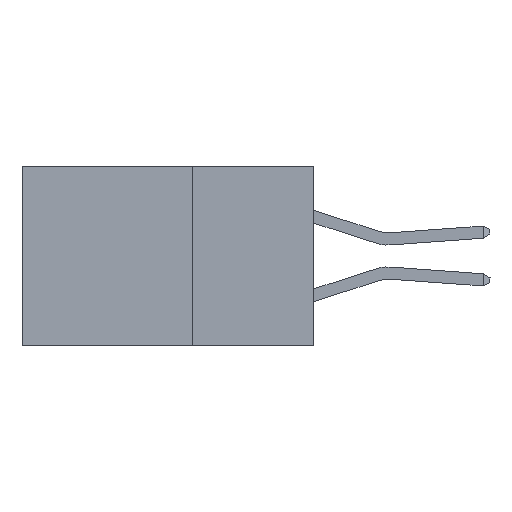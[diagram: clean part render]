
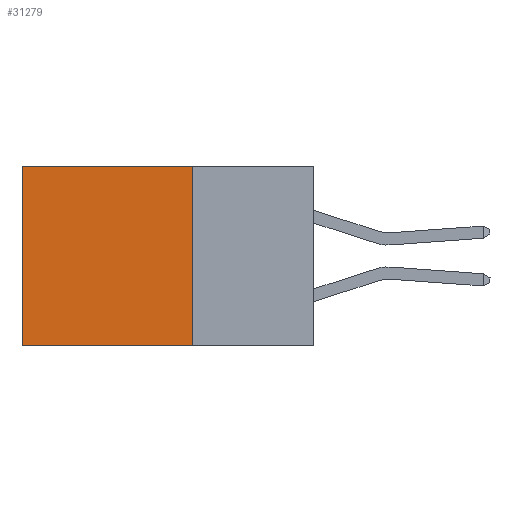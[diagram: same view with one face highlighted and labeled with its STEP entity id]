
A CAD part, left-side view. The second image highlights one B-rep face of the part: STEP entity #31279.
In plain terms, the highlighted planar face has unit normal (-1, 0, 0).
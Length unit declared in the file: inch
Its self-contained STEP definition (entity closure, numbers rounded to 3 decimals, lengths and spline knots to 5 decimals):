
#3481 = DIRECTION ( 'NONE',  ( 0., 1., 0. ) ) ;
#3822 = AXIS2_PLACEMENT_3D ( 'NONE', #17854, #40939, #38751 ) ;
#3990 = VECTOR ( 'NONE', #18243, 39.37008 ) ;
#4964 = VERTEX_POINT ( 'NONE', #37860 ) ;
#6355 = VERTEX_POINT ( 'NONE', #9526 ) ;
#9027 = ORIENTED_EDGE ( 'NONE', *, *, #21000, .T. ) ;
#9526 = CARTESIAN_POINT ( 'NONE',  ( 0.2875, 0.25, -0.37 ) ) ;
#10712 = LINE ( 'NONE', #21276, #3990 ) ;
#11021 = CARTESIAN_POINT ( 'NONE',  ( 0.2875, 0.25, 0. ) ) ;
#11824 = LINE ( 'NONE', #33800, #39691 ) ;
#13822 = LINE ( 'NONE', #11021, #35993 ) ;
#14432 = EDGE_CURVE ( 'NONE', #6355, #21913, #11824, .T. ) ;
#17854 = CARTESIAN_POINT ( 'NONE',  ( 0.2875, 0.25, 0. ) ) ;
#18048 = EDGE_CURVE ( 'NONE', #4964, #6355, #41953, .T. ) ;
#18168 = DIRECTION ( 'NONE',  ( 0., 0., -1. ) ) ;
#18243 = DIRECTION ( 'NONE',  ( 0., 0., -1. ) ) ;
#19058 = CARTESIAN_POINT ( 'NONE',  ( 0.2875, 0.6, -0.37 ) ) ;
#19854 = ORIENTED_EDGE ( 'NONE', *, *, #21132, .T. ) ;
#19924 = ORIENTED_EDGE ( 'NONE', *, *, #18048, .F. ) ;
#20556 = DIRECTION ( 'NONE',  ( 0., 1., 0. ) ) ;
#21000 = EDGE_CURVE ( 'NONE', #4964, #30920, #13822, .T. ) ;
#21132 = EDGE_CURVE ( 'NONE', #30920, #21913, #10712, .T. ) ;
#21276 = CARTESIAN_POINT ( 'NONE',  ( 0.2875, 0.6, 0. ) ) ;
#21617 = CARTESIAN_POINT ( 'NONE',  ( 0.2875, 0.25, 0. ) ) ;
#21913 = VERTEX_POINT ( 'NONE', #19058 ) ;
#28773 = EDGE_LOOP ( 'NONE', ( #19854, #35651, #19924, #9027 ) ) ;
#28971 = FACE_OUTER_BOUND ( 'NONE', #28773, .T. ) ;
#30920 = VERTEX_POINT ( 'NONE', #36635 ) ;
#31123 = VECTOR ( 'NONE', #18168, 39.37008 ) ;
#31279 = ADVANCED_FACE ( 'NONE', ( #28971 ), #37625, .F. ) ;
#33800 = CARTESIAN_POINT ( 'NONE',  ( 0.2875, 0.25, -0.37 ) ) ;
#35651 = ORIENTED_EDGE ( 'NONE', *, *, #14432, .F. ) ;
#35993 = VECTOR ( 'NONE', #20556, 39.37008 ) ;
#36635 = CARTESIAN_POINT ( 'NONE',  ( 0.2875, 0.6, 0. ) ) ;
#37625 = PLANE ( 'NONE',  #3822 ) ;
#37860 = CARTESIAN_POINT ( 'NONE',  ( 0.2875, 0.25, 0. ) ) ;
#38751 = DIRECTION ( 'NONE',  ( 0., 0., -1. ) ) ;
#39691 = VECTOR ( 'NONE', #3481, 39.37008 ) ;
#40939 = DIRECTION ( 'NONE',  ( 1., 0., 0. ) ) ;
#41953 = LINE ( 'NONE', #21617, #31123 ) ;
